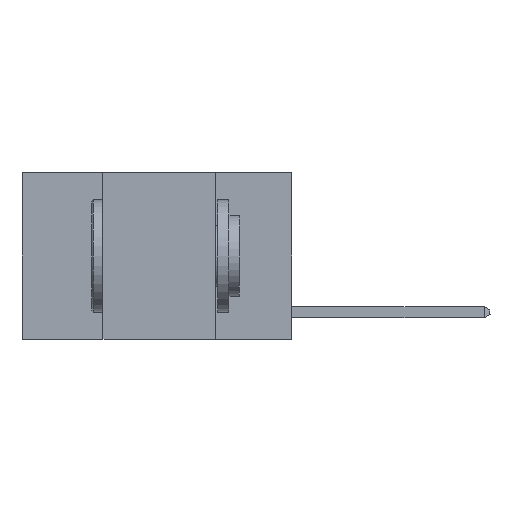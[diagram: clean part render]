
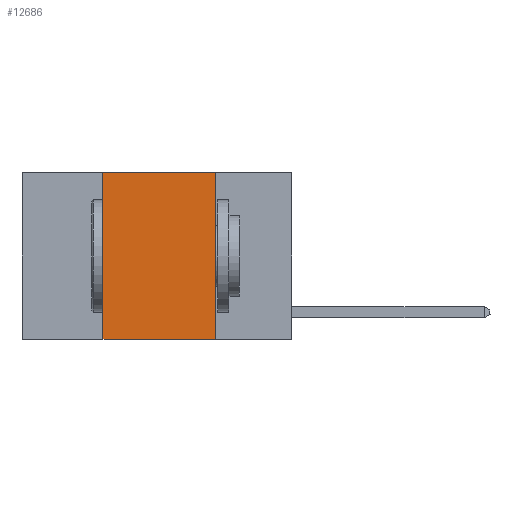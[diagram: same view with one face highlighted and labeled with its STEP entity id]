
A CAD part, left-side view. The second image highlights one B-rep face of the part: STEP entity #12686.
In plain terms, the highlighted planar face has unit normal (-1, 0, 0).
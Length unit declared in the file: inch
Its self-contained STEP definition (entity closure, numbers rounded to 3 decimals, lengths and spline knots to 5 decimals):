
#116 = VERTEX_POINT ( 'NONE', #8543 ) ;
#1082 = DIRECTION ( 'NONE',  ( 0., 0., -1. ) ) ;
#1346 = LINE ( 'NONE', #3474, #24720 ) ;
#2350 = DIRECTION ( 'NONE',  ( 0., -1., 0. ) ) ;
#2885 = DIRECTION ( 'NONE',  ( 0., -1., 0. ) ) ;
#3061 = CARTESIAN_POINT ( 'NONE',  ( 0., 0.17, 0. ) ) ;
#3474 = CARTESIAN_POINT ( 'NONE',  ( 0., 0.42, 0. ) ) ;
#4360 = LINE ( 'NONE', #10712, #15972 ) ;
#4878 = CARTESIAN_POINT ( 'NONE',  ( 0., 0.6, -0.37 ) ) ;
#5742 = EDGE_CURVE ( 'NONE', #26220, #11527, #23473, .T. ) ;
#7575 = ORIENTED_EDGE ( 'NONE', *, *, #17192, .F. ) ;
#7773 = DIRECTION ( 'NONE',  ( 0., 0., 1. ) ) ;
#8347 = ORIENTED_EDGE ( 'NONE', *, *, #17317, .F. ) ;
#8543 = CARTESIAN_POINT ( 'NONE',  ( 0., 0.42, 0. ) ) ;
#9965 = CARTESIAN_POINT ( 'NONE',  ( 0., 0.17, 0. ) ) ;
#10712 = CARTESIAN_POINT ( 'NONE',  ( 0., 0.6, 0. ) ) ;
#11301 = AXIS2_PLACEMENT_3D ( 'NONE', #16070, #16217, #24396 ) ;
#11527 = VERTEX_POINT ( 'NONE', #12263 ) ;
#12263 = CARTESIAN_POINT ( 'NONE',  ( 0., 0.17, -0.37 ) ) ;
#12686 = ADVANCED_FACE ( 'NONE', ( #18052 ), #26104, .F. ) ;
#13533 = VERTEX_POINT ( 'NONE', #9965 ) ;
#15000 = CARTESIAN_POINT ( 'NONE',  ( 0., 0.42, -0.37 ) ) ;
#15972 = VECTOR ( 'NONE', #2350, 39.37008 ) ;
#16070 = CARTESIAN_POINT ( 'NONE',  ( 0., 0.6, 0. ) ) ;
#16142 = ORIENTED_EDGE ( 'NONE', *, *, #21811, .F. ) ;
#16217 = DIRECTION ( 'NONE',  ( 1., 0., 0. ) ) ;
#17192 = EDGE_CURVE ( 'NONE', #13533, #11527, #21407, .T. ) ;
#17317 = EDGE_CURVE ( 'NONE', #26220, #116, #1346, .T. ) ;
#18052 = FACE_OUTER_BOUND ( 'NONE', #25976, .T. ) ;
#21407 = LINE ( 'NONE', #3061, #23036 ) ;
#21811 = EDGE_CURVE ( 'NONE', #116, #13533, #4360, .T. ) ;
#23036 = VECTOR ( 'NONE', #1082, 39.37008 ) ;
#23473 = LINE ( 'NONE', #4878, #25920 ) ;
#24396 = DIRECTION ( 'NONE',  ( 0., 0., -1. ) ) ;
#24720 = VECTOR ( 'NONE', #7773, 39.37008 ) ;
#24855 = ORIENTED_EDGE ( 'NONE', *, *, #5742, .T. ) ;
#25920 = VECTOR ( 'NONE', #2885, 39.37008 ) ;
#25976 = EDGE_LOOP ( 'NONE', ( #7575, #16142, #8347, #24855 ) ) ;
#26104 = PLANE ( 'NONE',  #11301 ) ;
#26220 = VERTEX_POINT ( 'NONE', #15000 ) ;
